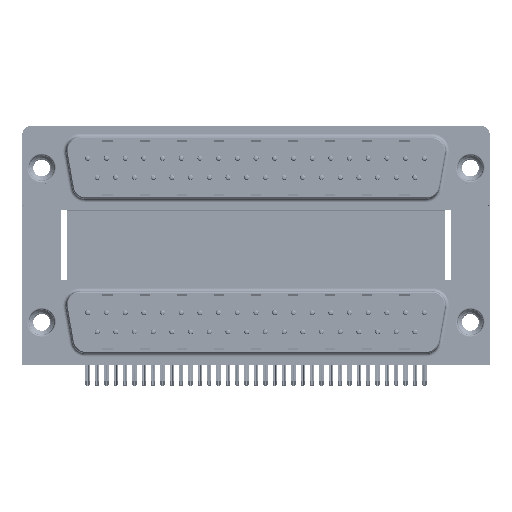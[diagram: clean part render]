
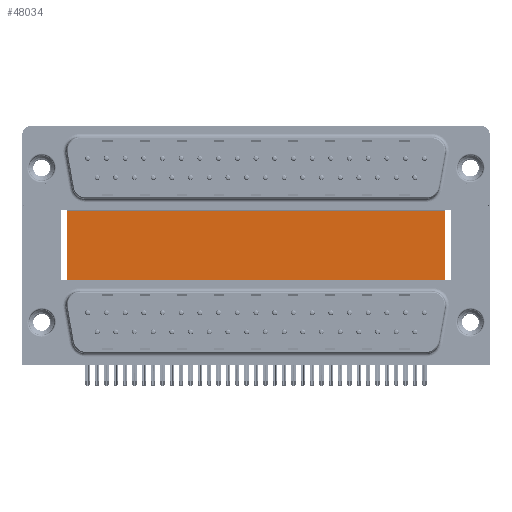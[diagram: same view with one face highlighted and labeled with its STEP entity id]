
A CAD part, top view. The second image highlights one B-rep face of the part: STEP entity #48034.
In plain terms, the highlighted planar face has unit normal (0, 0, 1).
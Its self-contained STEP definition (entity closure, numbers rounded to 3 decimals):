
#14 = CARTESIAN_POINT ( 'NONE',  ( 59.71, -3.735, -12. ) ) ;
#2139 = VERTEX_POINT ( 'NONE', #38357 ) ;
#2281 = LINE ( 'NONE', #5389, #34777 ) ;
#3954 = PLANE ( 'NONE',  #22375 ) ;
#4156 = VERTEX_POINT ( 'NONE', #21137 ) ;
#4563 = LINE ( 'NONE', #24129, #22713 ) ;
#5389 = CARTESIAN_POINT ( 'NONE',  ( 3.79, 16.585, -12. ) ) ;
#8858 = VECTOR ( 'NONE', #47947, 1000. ) ;
#9273 = EDGE_LOOP ( 'NONE', ( #47205, #43061, #15051, #18021 ) ) ;
#11872 = VECTOR ( 'NONE', #33558, 1000. ) ;
#15051 = ORIENTED_EDGE ( 'NONE', *, *, #42721, .F. ) ;
#15544 = CARTESIAN_POINT ( 'NONE',  ( 3.79, 16.585, -12. ) ) ;
#17289 = EDGE_CURVE ( 'NONE', #34012, #4156, #2281, .T. ) ;
#18021 = ORIENTED_EDGE ( 'NONE', *, *, #17289, .T. ) ;
#18401 = EDGE_CURVE ( 'NONE', #2139, #18516, #23708, .T. ) ;
#18516 = VERTEX_POINT ( 'NONE', #14 ) ;
#20279 = DIRECTION ( 'NONE',  ( 1., 0., 0. ) ) ;
#20320 = CARTESIAN_POINT ( 'NONE',  ( 3.79, 16.585, -12. ) ) ;
#21137 = CARTESIAN_POINT ( 'NONE',  ( 3.79, -3.735, -12. ) ) ;
#22375 = AXIS2_PLACEMENT_3D ( 'NONE', #15544, #47187, #26626 ) ;
#22713 = VECTOR ( 'NONE', #20279, 1000. ) ;
#23708 = LINE ( 'NONE', #47113, #11872 ) ;
#24129 = CARTESIAN_POINT ( 'NONE',  ( 3.79, -3.735, -12. ) ) ;
#24792 = LINE ( 'NONE', #34933, #8858 ) ;
#26626 = DIRECTION ( 'NONE',  ( -1., 0., 0. ) ) ;
#33558 = DIRECTION ( 'NONE',  ( 0., -1., 0. ) ) ;
#34012 = VERTEX_POINT ( 'NONE', #20320 ) ;
#34777 = VECTOR ( 'NONE', #37286, 1000. ) ;
#34933 = CARTESIAN_POINT ( 'NONE',  ( 3.79, 16.585, -12. ) ) ;
#35742 = EDGE_CURVE ( 'NONE', #4156, #18516, #4563, .T. ) ;
#37286 = DIRECTION ( 'NONE',  ( 0., -1., 0. ) ) ;
#38357 = CARTESIAN_POINT ( 'NONE',  ( 59.71, 16.585, -12. ) ) ;
#39209 = FACE_OUTER_BOUND ( 'NONE', #9273, .T. ) ;
#42721 = EDGE_CURVE ( 'NONE', #34012, #2139, #24792, .T. ) ;
#43061 = ORIENTED_EDGE ( 'NONE', *, *, #18401, .F. ) ;
#47113 = CARTESIAN_POINT ( 'NONE',  ( 59.71, 16.585, -12. ) ) ;
#47187 = DIRECTION ( 'NONE',  ( 0., 0., -1. ) ) ;
#47205 = ORIENTED_EDGE ( 'NONE', *, *, #35742, .T. ) ;
#47947 = DIRECTION ( 'NONE',  ( 1., 0., 0. ) ) ;
#48034 = ADVANCED_FACE ( 'NONE', ( #39209 ), #3954, .F. ) ;
